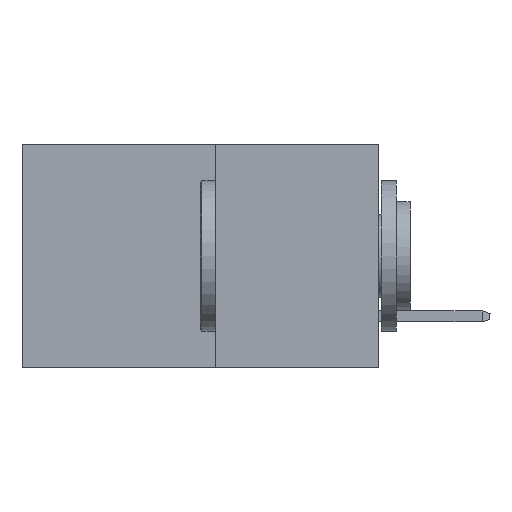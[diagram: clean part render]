
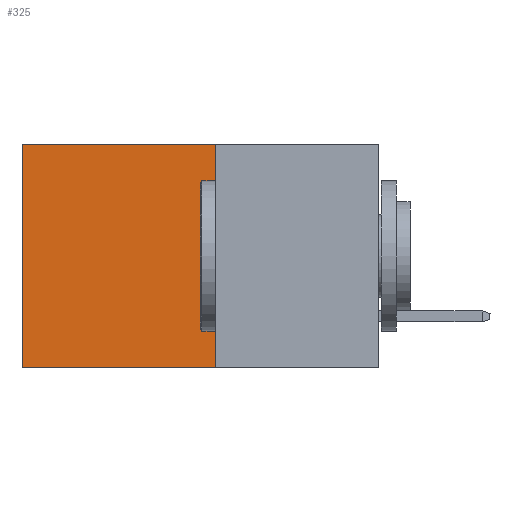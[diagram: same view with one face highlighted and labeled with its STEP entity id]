
A CAD part, left-side view. The second image highlights one B-rep face of the part: STEP entity #325.
In plain terms, the highlighted planar face has unit normal (-1, 0, 0).
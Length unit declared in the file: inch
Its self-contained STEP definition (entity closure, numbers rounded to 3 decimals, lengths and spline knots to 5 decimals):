
#254 = VECTOR ( 'NONE', #6078, 39.37008 ) ;
#325 = ADVANCED_FACE ( 'NONE', ( #7490 ), #2134, .F. ) ;
#1283 = DIRECTION ( 'NONE',  ( 0., 0., -1. ) ) ;
#1485 = ORIENTED_EDGE ( 'NONE', *, *, #5179, .F. ) ;
#1490 = VECTOR ( 'NONE', #3636, 39.37008 ) ;
#2134 = PLANE ( 'NONE',  #3099 ) ;
#2236 = VECTOR ( 'NONE', #13929, 39.37008 ) ;
#2660 = EDGE_CURVE ( 'NONE', #11842, #12740, #15199, .T. ) ;
#3099 = AXIS2_PLACEMENT_3D ( 'NONE', #15470, #14984, #1283 ) ;
#3419 = VECTOR ( 'NONE', #6256, 39.37008 ) ;
#3636 = DIRECTION ( 'NONE',  ( 0., 0., -1. ) ) ;
#3765 = CARTESIAN_POINT ( 'NONE',  ( 0.277, 0.27, -0.37 ) ) ;
#4911 = LINE ( 'NONE', #7353, #1490 ) ;
#5179 = EDGE_CURVE ( 'NONE', #15275, #12740, #6769, .T. ) ;
#5338 = CARTESIAN_POINT ( 'NONE',  ( 0.277, 0.27, 0. ) ) ;
#5935 = CARTESIAN_POINT ( 'NONE',  ( 0.277, 0.27, -0.37 ) ) ;
#6078 = DIRECTION ( 'NONE',  ( 0., 1., 0. ) ) ;
#6256 = DIRECTION ( 'NONE',  ( 0., 1., 0. ) ) ;
#6769 = LINE ( 'NONE', #5935, #3419 ) ;
#7166 = CARTESIAN_POINT ( 'NONE',  ( 0.277, 0.59, -0.37 ) ) ;
#7353 = CARTESIAN_POINT ( 'NONE',  ( 0.277, 0.27, -0.37 ) ) ;
#7490 = FACE_OUTER_BOUND ( 'NONE', #10665, .T. ) ;
#7813 = ORIENTED_EDGE ( 'NONE', *, *, #2660, .T. ) ;
#8156 = EDGE_CURVE ( 'NONE', #8448, #15275, #4911, .T. ) ;
#8448 = VERTEX_POINT ( 'NONE', #5338 ) ;
#8515 = CARTESIAN_POINT ( 'NONE',  ( 0.277, 0.59, 0. ) ) ;
#10665 = EDGE_LOOP ( 'NONE', ( #7813, #1485, #11589, #11959 ) ) ;
#11589 = ORIENTED_EDGE ( 'NONE', *, *, #8156, .F. ) ;
#11842 = VERTEX_POINT ( 'NONE', #8515 ) ;
#11959 = ORIENTED_EDGE ( 'NONE', *, *, #13549, .T. ) ;
#12740 = VERTEX_POINT ( 'NONE', #7166 ) ;
#12986 = CARTESIAN_POINT ( 'NONE',  ( 0.277, 0.27, 0. ) ) ;
#13197 = LINE ( 'NONE', #12986, #254 ) ;
#13549 = EDGE_CURVE ( 'NONE', #8448, #11842, #13197, .T. ) ;
#13929 = DIRECTION ( 'NONE',  ( 0., 0., -1. ) ) ;
#14055 = CARTESIAN_POINT ( 'NONE',  ( 0.277, 0.59, -0.37 ) ) ;
#14984 = DIRECTION ( 'NONE',  ( 1., 0., 0. ) ) ;
#15199 = LINE ( 'NONE', #14055, #2236 ) ;
#15275 = VERTEX_POINT ( 'NONE', #3765 ) ;
#15470 = CARTESIAN_POINT ( 'NONE',  ( 0.277, 0.27, -0.37 ) ) ;
